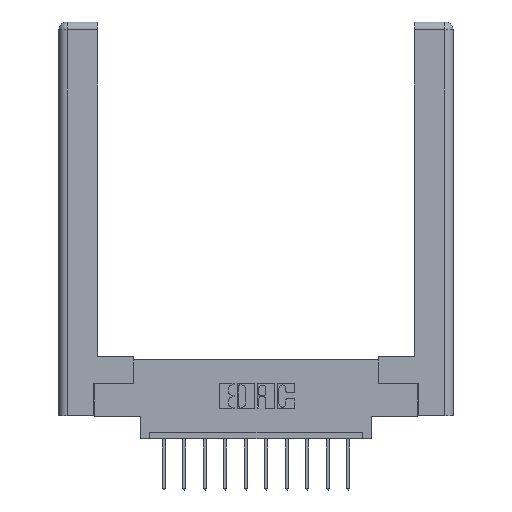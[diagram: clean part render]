
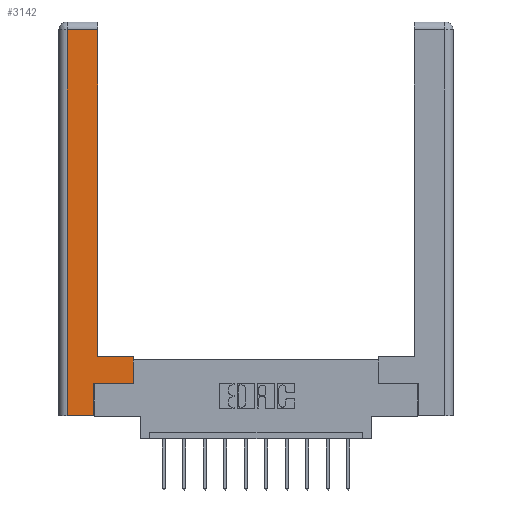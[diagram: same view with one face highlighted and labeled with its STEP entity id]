
A CAD part, top view. The second image highlights one B-rep face of the part: STEP entity #3142.
In plain terms, the highlighted planar face has unit normal (0, 0, 1).
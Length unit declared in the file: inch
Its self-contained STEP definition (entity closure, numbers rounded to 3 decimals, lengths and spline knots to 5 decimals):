
#34 = VERTEX_POINT ( 'NONE', #8960 ) ;
#546 = LINE ( 'NONE', #908, #10634 ) ;
#565 = CARTESIAN_POINT ( 'NONE',  ( 0.265, 0.245, 0. ) ) ;
#750 = ORIENTED_EDGE ( 'NONE', *, *, #8281, .T. ) ;
#908 = CARTESIAN_POINT ( 'NONE',  ( 0.565, 0.45, 0. ) ) ;
#1295 = VERTEX_POINT ( 'NONE', #8545 ) ;
#1388 = LINE ( 'NONE', #9428, #12325 ) ;
#1610 = ORIENTED_EDGE ( 'NONE', *, *, #2221, .T. ) ;
#2221 = EDGE_CURVE ( 'NONE', #8015, #1295, #3940, .T. ) ;
#3142 = ADVANCED_FACE ( 'NONE', ( #8912 ), #5613, .F. ) ;
#3166 = LINE ( 'NONE', #14061, #9060 ) ;
#3223 = CARTESIAN_POINT ( 'NONE',  ( 0., 0., 0. ) ) ;
#3581 = ORIENTED_EDGE ( 'NONE', *, *, #14009, .T. ) ;
#3740 = DIRECTION ( 'NONE',  ( -1., 0., 0. ) ) ;
#3940 = LINE ( 'NONE', #4685, #11377 ) ;
#4685 = CARTESIAN_POINT ( 'NONE',  ( 0.295, 0.45, 0. ) ) ;
#4853 = CARTESIAN_POINT ( 'NONE',  ( 0.0615, 0., 0. ) ) ;
#4887 = EDGE_CURVE ( 'NONE', #12900, #9427, #14302, .T. ) ;
#5029 = LINE ( 'NONE', #11378, #6234 ) ;
#5247 = ORIENTED_EDGE ( 'NONE', *, *, #9508, .T. ) ;
#5327 = DIRECTION ( 'NONE',  ( -1., 0., 0. ) ) ;
#5613 = PLANE ( 'NONE',  #8903 ) ;
#5819 = CARTESIAN_POINT ( 'NONE',  ( 0.565, 0.245, 0. ) ) ;
#5870 = VECTOR ( 'NONE', #5327, 39.37008 ) ;
#6146 = ORIENTED_EDGE ( 'NONE', *, *, #14169, .T. ) ;
#6234 = VECTOR ( 'NONE', #12522, 39.37008 ) ;
#6522 = EDGE_CURVE ( 'NONE', #9427, #8015, #546, .T. ) ;
#6642 = ORIENTED_EDGE ( 'NONE', *, *, #13790, .T. ) ;
#6643 = ORIENTED_EDGE ( 'NONE', *, *, #6522, .T. ) ;
#6981 = CARTESIAN_POINT ( 'NONE',  ( 0.565, 0.45, 0. ) ) ;
#7144 = DIRECTION ( 'NONE',  ( 0., -1., 0. ) ) ;
#7693 = VECTOR ( 'NONE', #13197, 39.37008 ) ;
#7787 = LINE ( 'NONE', #9871, #5870 ) ;
#7931 = CARTESIAN_POINT ( 'NONE',  ( 0.0615, 2.94, 0. ) ) ;
#8015 = VERTEX_POINT ( 'NONE', #6981 ) ;
#8281 = EDGE_CURVE ( 'NONE', #34, #12900, #3166, .T. ) ;
#8545 = CARTESIAN_POINT ( 'NONE',  ( 0.295, 0.45, 0. ) ) ;
#8670 = VERTEX_POINT ( 'NONE', #7931 ) ;
#8877 = DIRECTION ( 'NONE',  ( 0., 0., -1. ) ) ;
#8903 = AXIS2_PLACEMENT_3D ( 'NONE', #3223, #8877, #9921 ) ;
#8912 = FACE_OUTER_BOUND ( 'NONE', #13425, .T. ) ;
#8960 = CARTESIAN_POINT ( 'NONE',  ( 0.265, 0., 0. ) ) ;
#9025 = ORIENTED_EDGE ( 'NONE', *, *, #4887, .T. ) ;
#9060 = VECTOR ( 'NONE', #10761, 39.37008 ) ;
#9427 = VERTEX_POINT ( 'NONE', #5819 ) ;
#9428 = CARTESIAN_POINT ( 'NONE',  ( 0.295, 3., 0. ) ) ;
#9508 = EDGE_CURVE ( 'NONE', #8670, #13998, #13535, .T. ) ;
#9871 = CARTESIAN_POINT ( 'NONE',  ( 0.0615, 2.94, 0. ) ) ;
#9911 = VECTOR ( 'NONE', #7144, 39.37008 ) ;
#9921 = DIRECTION ( 'NONE',  ( -1., 0., 0. ) ) ;
#10425 = VERTEX_POINT ( 'NONE', #12075 ) ;
#10634 = VECTOR ( 'NONE', #14252, 39.37008 ) ;
#10761 = DIRECTION ( 'NONE',  ( 0., 1., 0. ) ) ;
#11377 = VECTOR ( 'NONE', #3740, 39.37008 ) ;
#11378 = CARTESIAN_POINT ( 'NONE',  ( 0.265, 0., 0. ) ) ;
#11774 = CARTESIAN_POINT ( 'NONE',  ( 0.0615, 0., 0. ) ) ;
#12075 = CARTESIAN_POINT ( 'NONE',  ( 0.295, 2.94, 0. ) ) ;
#12234 = CARTESIAN_POINT ( 'NONE',  ( 0.565, 0.245, 0. ) ) ;
#12325 = VECTOR ( 'NONE', #14025, 39.37008 ) ;
#12522 = DIRECTION ( 'NONE',  ( 1., 0., 0. ) ) ;
#12900 = VERTEX_POINT ( 'NONE', #565 ) ;
#13197 = DIRECTION ( 'NONE',  ( 1., 0., 0. ) ) ;
#13425 = EDGE_LOOP ( 'NONE', ( #3581, #6146, #5247, #6642, #750, #9025, #6643, #1610 ) ) ;
#13535 = LINE ( 'NONE', #11774, #9911 ) ;
#13790 = EDGE_CURVE ( 'NONE', #13998, #34, #5029, .T. ) ;
#13998 = VERTEX_POINT ( 'NONE', #4853 ) ;
#14009 = EDGE_CURVE ( 'NONE', #1295, #10425, #1388, .T. ) ;
#14025 = DIRECTION ( 'NONE',  ( 0., 1., 0. ) ) ;
#14061 = CARTESIAN_POINT ( 'NONE',  ( 0.265, 0.245, 0. ) ) ;
#14169 = EDGE_CURVE ( 'NONE', #10425, #8670, #7787, .T. ) ;
#14252 = DIRECTION ( 'NONE',  ( 0., 1., 0. ) ) ;
#14302 = LINE ( 'NONE', #12234, #7693 ) ;
